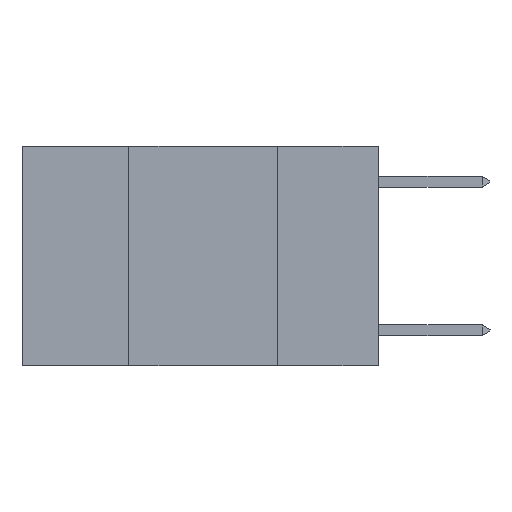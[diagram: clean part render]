
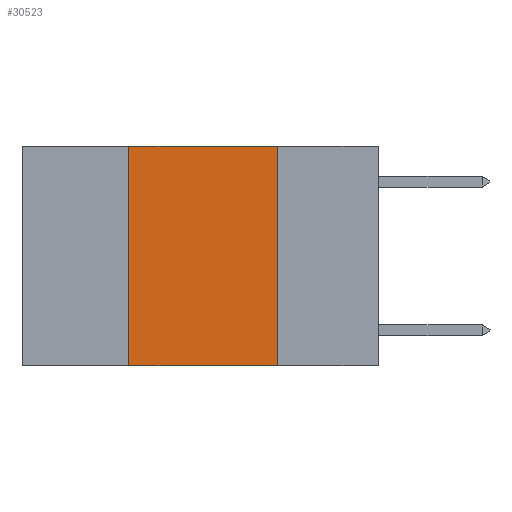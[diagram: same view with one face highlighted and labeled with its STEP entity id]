
A CAD part, left-side view. The second image highlights one B-rep face of the part: STEP entity #30523.
In plain terms, the highlighted planar face has unit normal (-1, 0, 0).
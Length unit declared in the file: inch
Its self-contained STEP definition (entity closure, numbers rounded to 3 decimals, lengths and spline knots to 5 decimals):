
#698 = LINE ( 'NONE', #8216, #1881 ) ;
#1416 = EDGE_CURVE ( 'NONE', #28113, #27179, #698, .T. ) ;
#1800 = CARTESIAN_POINT ( 'NONE',  ( 0., 0.6, -0.37 ) ) ;
#1881 = VECTOR ( 'NONE', #5550, 39.37008 ) ;
#3535 = DIRECTION ( 'NONE',  ( 0., 0., -1. ) ) ;
#3856 = DIRECTION ( 'NONE',  ( 1., 0., 0. ) ) ;
#5550 = DIRECTION ( 'NONE',  ( 0., 0., -1. ) ) ;
#7070 = VECTOR ( 'NONE', #28687, 39.37008 ) ;
#8205 = VERTEX_POINT ( 'NONE', #21524 ) ;
#8216 = CARTESIAN_POINT ( 'NONE',  ( 0., 0.17, 0. ) ) ;
#8873 = PLANE ( 'NONE',  #18239 ) ;
#11137 = EDGE_CURVE ( 'NONE', #8205, #27179, #23069, .T. ) ;
#12456 = CARTESIAN_POINT ( 'NONE',  ( 0., 0.42, 0. ) ) ;
#12877 = VECTOR ( 'NONE', #31032, 39.37008 ) ;
#13132 = LINE ( 'NONE', #18493, #7070 ) ;
#13974 = ORIENTED_EDGE ( 'NONE', *, *, #1416, .F. ) ;
#14661 = ORIENTED_EDGE ( 'NONE', *, *, #11137, .T. ) ;
#15012 = ORIENTED_EDGE ( 'NONE', *, *, #23699, .F. ) ;
#15222 = EDGE_LOOP ( 'NONE', ( #13974, #15012, #20374, #14661 ) ) ;
#16258 = FACE_OUTER_BOUND ( 'NONE', #15222, .T. ) ;
#18239 = AXIS2_PLACEMENT_3D ( 'NONE', #31462, #3856, #3535 ) ;
#18250 = CARTESIAN_POINT ( 'NONE',  ( 0., 0.17, -0.37 ) ) ;
#18493 = CARTESIAN_POINT ( 'NONE',  ( 0., 0.6, 0. ) ) ;
#20374 = ORIENTED_EDGE ( 'NONE', *, *, #22337, .F. ) ;
#21315 = LINE ( 'NONE', #28681, #12877 ) ;
#21524 = CARTESIAN_POINT ( 'NONE',  ( 0., 0.42, -0.37 ) ) ;
#22337 = EDGE_CURVE ( 'NONE', #8205, #31790, #21315, .T. ) ;
#23069 = LINE ( 'NONE', #1800, #28010 ) ;
#23699 = EDGE_CURVE ( 'NONE', #31790, #28113, #13132, .T. ) ;
#25864 = CARTESIAN_POINT ( 'NONE',  ( 0., 0.17, 0. ) ) ;
#27179 = VERTEX_POINT ( 'NONE', #18250 ) ;
#28010 = VECTOR ( 'NONE', #30262, 39.37008 ) ;
#28113 = VERTEX_POINT ( 'NONE', #25864 ) ;
#28681 = CARTESIAN_POINT ( 'NONE',  ( 0., 0.42, 0. ) ) ;
#28687 = DIRECTION ( 'NONE',  ( 0., -1., 0. ) ) ;
#30262 = DIRECTION ( 'NONE',  ( 0., -1., 0. ) ) ;
#30523 = ADVANCED_FACE ( 'NONE', ( #16258 ), #8873, .F. ) ;
#31032 = DIRECTION ( 'NONE',  ( 0., 0., 1. ) ) ;
#31462 = CARTESIAN_POINT ( 'NONE',  ( 0., 0.6, 0. ) ) ;
#31790 = VERTEX_POINT ( 'NONE', #12456 ) ;
